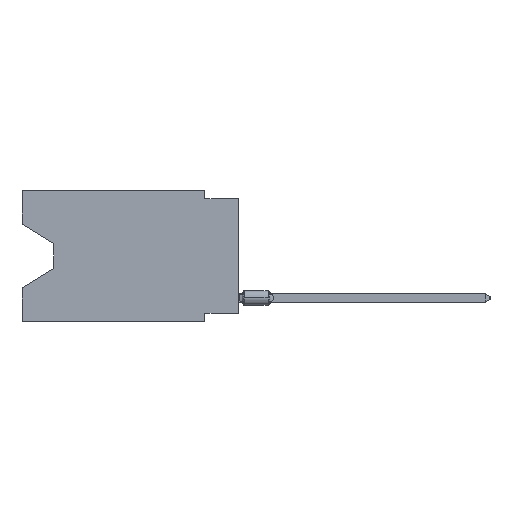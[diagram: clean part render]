
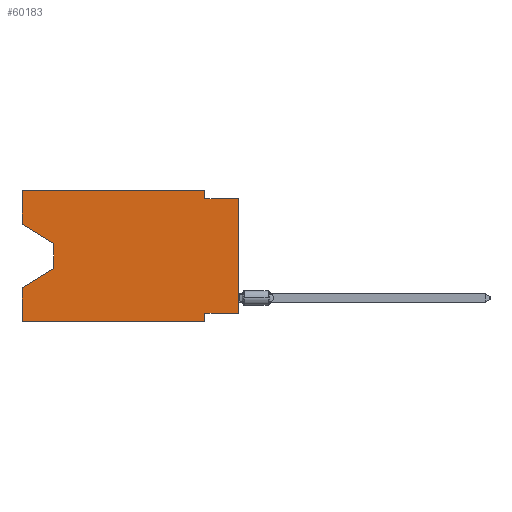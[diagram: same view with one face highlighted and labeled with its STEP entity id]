
A CAD part, left-side view. The second image highlights one B-rep face of the part: STEP entity #60183.
In plain terms, the highlighted planar face has unit normal (-1, 0, 0).
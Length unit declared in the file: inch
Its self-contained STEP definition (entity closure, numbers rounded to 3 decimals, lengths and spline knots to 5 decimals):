
#140 = VECTOR ( 'NONE', #27606, 39.37008 ) ;
#509 = VECTOR ( 'NONE', #7975, 39.37008 ) ;
#1347 = VECTOR ( 'NONE', #65902, 39.37008 ) ;
#1365 = CARTESIAN_POINT ( 'NONE',  ( 0., 0.1, -0.365 ) ) ;
#1410 = VERTEX_POINT ( 'NONE', #37077 ) ;
#2543 = CARTESIAN_POINT ( 'NONE',  ( 0., 0.55, -0.232 ) ) ;
#2670 = LINE ( 'NONE', #65905, #9269 ) ;
#2988 = ORIENTED_EDGE ( 'NONE', *, *, #60961, .T. ) ;
#4206 = ORIENTED_EDGE ( 'NONE', *, *, #40067, .T. ) ;
#4250 = VERTEX_POINT ( 'NONE', #22311 ) ;
#4535 = VECTOR ( 'NONE', #29882, 39.37008 ) ;
#6429 = DIRECTION ( 'NONE',  ( 0., 0., -1. ) ) ;
#7975 = DIRECTION ( 'NONE',  ( 0., -1., 0. ) ) ;
#8386 = EDGE_CURVE ( 'NONE', #48198, #58415, #70316, .T. ) ;
#8653 = VERTEX_POINT ( 'NONE', #69762 ) ;
#9269 = VECTOR ( 'NONE', #25658, 39.37008 ) ;
#9719 = CARTESIAN_POINT ( 'NONE',  ( 0., 0.645, 0. ) ) ;
#9875 = VERTEX_POINT ( 'NONE', #64941 ) ;
#10245 = DIRECTION ( 'NONE',  ( 0., 1., 0. ) ) ;
#10610 = LINE ( 'NONE', #40353, #14417 ) ;
#11965 = EDGE_CURVE ( 'NONE', #1410, #48198, #45971, .T. ) ;
#13032 = CARTESIAN_POINT ( 'NONE',  ( 0., 0.1, 0. ) ) ;
#13897 = DIRECTION ( 'NONE',  ( 0., 0., -1. ) ) ;
#14417 = VECTOR ( 'NONE', #10245, 39.37008 ) ;
#15572 = VERTEX_POINT ( 'NONE', #23898 ) ;
#16102 = ORIENTED_EDGE ( 'NONE', *, *, #59131, .F. ) ;
#16155 = ORIENTED_EDGE ( 'NONE', *, *, #66915, .F. ) ;
#17454 = LINE ( 'NONE', #18199, #4535 ) ;
#18199 = CARTESIAN_POINT ( 'NONE',  ( 0., 0.1, -0.39 ) ) ;
#18486 = ORIENTED_EDGE ( 'NONE', *, *, #27242, .F. ) ;
#19550 = CARTESIAN_POINT ( 'NONE',  ( 0., 0.1, -0.025 ) ) ;
#20289 = FACE_OUTER_BOUND ( 'NONE', #57077, .T. ) ;
#20494 = DIRECTION ( 'NONE',  ( 0., 0., 1. ) ) ;
#21858 = CARTESIAN_POINT ( 'NONE',  ( 0., 0., 0. ) ) ;
#22311 = CARTESIAN_POINT ( 'NONE',  ( 0., 0.1, -0.39 ) ) ;
#22623 = AXIS2_PLACEMENT_3D ( 'NONE', #9719, #42874, #13897 ) ;
#23295 = EDGE_CURVE ( 'NONE', #8653, #53129, #2670, .T. ) ;
#23898 = CARTESIAN_POINT ( 'NONE',  ( 0., 0., -0.365 ) ) ;
#24131 = CARTESIAN_POINT ( 'NONE',  ( 0., 0.55, -0.158 ) ) ;
#24956 = ORIENTED_EDGE ( 'NONE', *, *, #8386, .T. ) ;
#25067 = VECTOR ( 'NONE', #43358, 39.37008 ) ;
#25658 = DIRECTION ( 'NONE',  ( 0., 0., 1. ) ) ;
#25841 = ORIENTED_EDGE ( 'NONE', *, *, #31286, .F. ) ;
#26339 = VERTEX_POINT ( 'NONE', #13032 ) ;
#26486 = DIRECTION ( 'NONE',  ( 0., -0.855, -0.519 ) ) ;
#26772 = CARTESIAN_POINT ( 'NONE',  ( 0., 0.645, -0.28975 ) ) ;
#27242 = EDGE_CURVE ( 'NONE', #58629, #59853, #70815, .T. ) ;
#27606 = DIRECTION ( 'NONE',  ( 0., -1., 0. ) ) ;
#29882 = DIRECTION ( 'NONE',  ( 0., 0., -1. ) ) ;
#29883 = EDGE_CURVE ( 'NONE', #8653, #1410, #43429, .T. ) ;
#31286 = EDGE_CURVE ( 'NONE', #53129, #26339, #65550, .T. ) ;
#32132 = CARTESIAN_POINT ( 'NONE',  ( 0., 0.645, -0.10025 ) ) ;
#32142 = CARTESIAN_POINT ( 'NONE',  ( 0., 0.645, -0.39 ) ) ;
#32437 = LINE ( 'NONE', #21858, #25067 ) ;
#32483 = VECTOR ( 'NONE', #42096, 39.37008 ) ;
#33133 = VERTEX_POINT ( 'NONE', #1365 ) ;
#33147 = ORIENTED_EDGE ( 'NONE', *, *, #38614, .F. ) ;
#34774 = ORIENTED_EDGE ( 'NONE', *, *, #29883, .T. ) ;
#35982 = ORIENTED_EDGE ( 'NONE', *, *, #57167, .F. ) ;
#36304 = ORIENTED_EDGE ( 'NONE', *, *, #11965, .T. ) ;
#36678 = CARTESIAN_POINT ( 'NONE',  ( 0., 0.55, -0.232 ) ) ;
#37077 = CARTESIAN_POINT ( 'NONE',  ( 0., 0.55, -0.158 ) ) ;
#38614 = EDGE_CURVE ( 'NONE', #15572, #33133, #10610, .T. ) ;
#40067 = EDGE_CURVE ( 'NONE', #9875, #4250, #43803, .T. ) ;
#40353 = CARTESIAN_POINT ( 'NONE',  ( 0., 0., -0.365 ) ) ;
#41489 = CARTESIAN_POINT ( 'NONE',  ( 0., 0.645, 0. ) ) ;
#42096 = DIRECTION ( 'NONE',  ( 0., 0.855, -0.519 ) ) ;
#42874 = DIRECTION ( 'NONE',  ( 1., 0., 0. ) ) ;
#43358 = DIRECTION ( 'NONE',  ( 0., 0., 1. ) ) ;
#43429 = LINE ( 'NONE', #32132, #66562 ) ;
#43455 = CARTESIAN_POINT ( 'NONE',  ( 0., 0.645, 0. ) ) ;
#43803 = LINE ( 'NONE', #32142, #140 ) ;
#45971 = LINE ( 'NONE', #24131, #60118 ) ;
#48198 = VERTEX_POINT ( 'NONE', #36678 ) ;
#51138 = VECTOR ( 'NONE', #61383, 39.37008 ) ;
#52100 = CARTESIAN_POINT ( 'NONE',  ( 0., 0.645, 0. ) ) ;
#53129 = VERTEX_POINT ( 'NONE', #52100 ) ;
#54619 = CARTESIAN_POINT ( 'NONE',  ( 0., 0., -0.025 ) ) ;
#55364 = LINE ( 'NONE', #61011, #51138 ) ;
#57077 = EDGE_LOOP ( 'NONE', ( #34774, #36304, #24956, #16102, #4206, #16155, #33147, #2988, #18486, #35982, #25841, #67900 ) ) ;
#57167 = EDGE_CURVE ( 'NONE', #26339, #58629, #55364, .T. ) ;
#58415 = VERTEX_POINT ( 'NONE', #26772 ) ;
#58629 = VERTEX_POINT ( 'NONE', #19550 ) ;
#59131 = EDGE_CURVE ( 'NONE', #9875, #58415, #72038, .T. ) ;
#59853 = VERTEX_POINT ( 'NONE', #68887 ) ;
#60118 = VECTOR ( 'NONE', #6429, 39.37008 ) ;
#60183 = ADVANCED_FACE ( 'NONE', ( #20289 ), #66929, .F. ) ;
#60961 = EDGE_CURVE ( 'NONE', #15572, #59853, #32437, .T. ) ;
#61011 = CARTESIAN_POINT ( 'NONE',  ( 0., 0.1, 0. ) ) ;
#61383 = DIRECTION ( 'NONE',  ( 0., 0., -1. ) ) ;
#62174 = VECTOR ( 'NONE', #20494, 39.37008 ) ;
#64941 = CARTESIAN_POINT ( 'NONE',  ( 0., 0.645, -0.39 ) ) ;
#65550 = LINE ( 'NONE', #41489, #509 ) ;
#65902 = DIRECTION ( 'NONE',  ( 0., -1., 0. ) ) ;
#65905 = CARTESIAN_POINT ( 'NONE',  ( 0., 0.645, 0. ) ) ;
#66562 = VECTOR ( 'NONE', #26486, 39.37008 ) ;
#66915 = EDGE_CURVE ( 'NONE', #33133, #4250, #17454, .T. ) ;
#66929 = PLANE ( 'NONE',  #22623 ) ;
#67900 = ORIENTED_EDGE ( 'NONE', *, *, #23295, .F. ) ;
#68887 = CARTESIAN_POINT ( 'NONE',  ( 0., 0., -0.025 ) ) ;
#69762 = CARTESIAN_POINT ( 'NONE',  ( 0., 0.645, -0.10025 ) ) ;
#70316 = LINE ( 'NONE', #2543, #32483 ) ;
#70815 = LINE ( 'NONE', #54619, #1347 ) ;
#72038 = LINE ( 'NONE', #43455, #62174 ) ;
